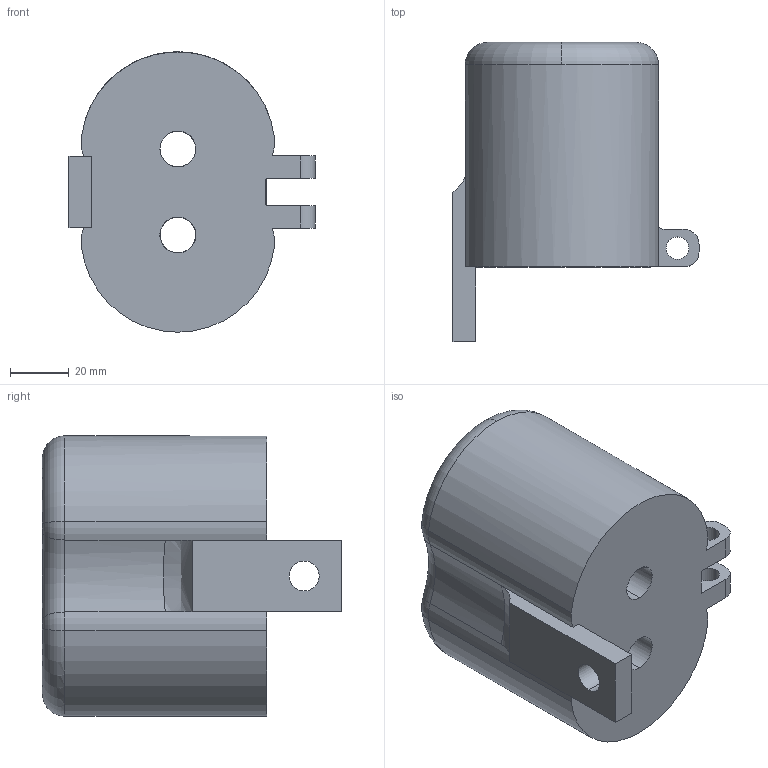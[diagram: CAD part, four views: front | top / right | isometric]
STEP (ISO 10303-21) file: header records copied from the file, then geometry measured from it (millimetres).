
FILE_DESCRIPTION (( 'STEP AP214' ), '1' );
FILE_NAME ('410barrel.STEP', '2013-07-25T16:59:43', ( '' ), ( '' ), 'SwSTEP 2.0', 'SolidWorks 2013', '' );
FILE_SCHEMA (( 'AUTOMOTIVE_DESIGN' ));
Length unit declared in the file: inch
Products named in the file (1): 410barrel
Bounding box: 83.56 x 101.6 x 95.24 mm (x, y, z)
Volume: 387181.1 mm3; surface area: 38761.5 mm2
Topology: 1 solids, 1 shells, 64 faces, 170 edges, 108 vertices
Faces by surface type: cylinder 31, torus 15, plane 15, bspline 3
Entity records: 3471 total; most frequent: CARTESIAN_POINT 1828, DIRECTION 349, ORIENTED_EDGE 340, EDGE_CURVE 170, AXIS2_PLACEMENT_3D 143, VERTEX_POINT 108, CIRCLE 81, EDGE_LOOP 74
